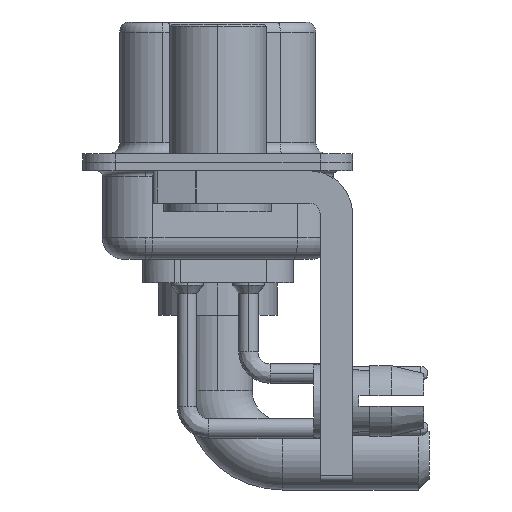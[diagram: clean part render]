
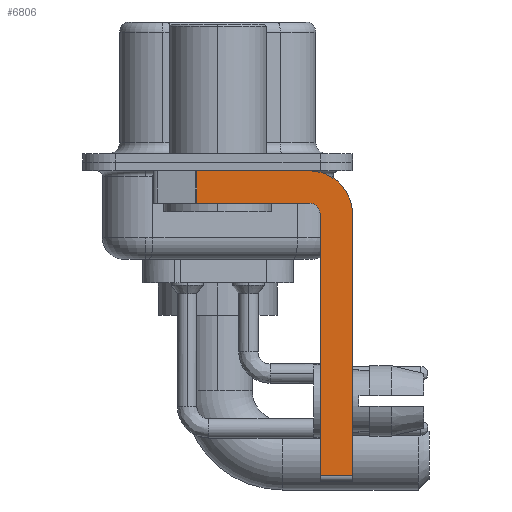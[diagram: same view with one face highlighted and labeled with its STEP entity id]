
A CAD part, left-side view. The second image highlights one B-rep face of the part: STEP entity #6806.
In plain terms, the highlighted planar face has unit normal (-1, 0, 0).
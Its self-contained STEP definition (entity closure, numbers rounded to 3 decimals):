
#232 = VERTEX_POINT ( 'NONE', #6532 ) ;
#1217 = CARTESIAN_POINT ( 'NONE',  ( -2.9, -4.75, -14.55 ) ) ;
#1303 = ORIENTED_EDGE ( 'NONE', *, *, #18957, .F. ) ;
#2598 = VERTEX_POINT ( 'NONE', #21329 ) ;
#3420 = LINE ( 'NONE', #29053, #27562 ) ;
#3523 = VECTOR ( 'NONE', #29938, 1000. ) ;
#3868 = DIRECTION ( 'NONE',  ( 0., 0., -1. ) ) ;
#3941 = DIRECTION ( 'NONE',  ( 0., 0., -1. ) ) ;
#4054 = DIRECTION ( 'NONE',  ( 1., 0., 0. ) ) ;
#4432 = LINE ( 'NONE', #11294, #3523 ) ;
#4617 = VECTOR ( 'NONE', #25354, 1000. ) ;
#4645 = CARTESIAN_POINT ( 'NONE',  ( -2.9, -4.25, -2.4 ) ) ;
#5770 = CARTESIAN_POINT ( 'NONE',  ( -2.9, -4.25, -2.4 ) ) ;
#5976 = AXIS2_PLACEMENT_3D ( 'NONE', #7387, #16223, #16380 ) ;
#6434 = EDGE_CURVE ( 'NONE', #29442, #24426, #17389, .T. ) ;
#6532 = CARTESIAN_POINT ( 'NONE',  ( -2.9, -4.25, -1.9 ) ) ;
#6806 = ADVANCED_FACE ( 'NONE', ( #10334 ), #15063, .F. ) ;
#6948 = VECTOR ( 'NONE', #23942, 1000. ) ;
#7024 = EDGE_CURVE ( 'NONE', #28893, #24217, #20632, .T. ) ;
#7387 = CARTESIAN_POINT ( 'NONE',  ( -2.9, -4.25, -2.4 ) ) ;
#8292 = ORIENTED_EDGE ( 'NONE', *, *, #28076, .F. ) ;
#9738 = ORIENTED_EDGE ( 'NONE', *, *, #29828, .T. ) ;
#9812 = ORIENTED_EDGE ( 'NONE', *, *, #18175, .F. ) ;
#10198 = EDGE_CURVE ( 'NONE', #14357, #15229, #3420, .T. ) ;
#10319 = ORIENTED_EDGE ( 'NONE', *, *, #6434, .F. ) ;
#10334 = FACE_OUTER_BOUND ( 'NONE', #21646, .T. ) ;
#10677 = CARTESIAN_POINT ( 'NONE',  ( -2.9, -4.75, -14.8 ) ) ;
#11294 = CARTESIAN_POINT ( 'NONE',  ( -2.9, -4.25, -1.9 ) ) ;
#12267 = CARTESIAN_POINT ( 'NONE',  ( -2.9, 3., -0.4 ) ) ;
#12476 = DIRECTION ( 'NONE',  ( 1., 0., 0. ) ) ;
#12500 = ORIENTED_EDGE ( 'NONE', *, *, #10198, .T. ) ;
#12681 = CARTESIAN_POINT ( 'NONE',  ( -2.9, 0.978, -0.4 ) ) ;
#14004 = CARTESIAN_POINT ( 'NONE',  ( -2.9, -4.75, -2.4 ) ) ;
#14151 = CARTESIAN_POINT ( 'NONE',  ( -2.9, 0.978, -1.9 ) ) ;
#14357 = VERTEX_POINT ( 'NONE', #12681 ) ;
#15063 = PLANE ( 'NONE',  #19733 ) ;
#15229 = VERTEX_POINT ( 'NONE', #14151 ) ;
#16108 = CARTESIAN_POINT ( 'NONE',  ( -2.9, -4.25, -14.55 ) ) ;
#16223 = DIRECTION ( 'NONE',  ( -1., 0., 0. ) ) ;
#16370 = ORIENTED_EDGE ( 'NONE', *, *, #7024, .F. ) ;
#16380 = DIRECTION ( 'NONE',  ( 0., 0., 1. ) ) ;
#17389 = LINE ( 'NONE', #10677, #26960 ) ;
#17644 = CIRCLE ( 'NONE', #5976, 0.5 ) ;
#17676 = DIRECTION ( 'NONE',  ( 0., 0., 1. ) ) ;
#17937 = CARTESIAN_POINT ( 'NONE',  ( -2.9, -6.25, -2.4 ) ) ;
#18000 = EDGE_CURVE ( 'NONE', #24426, #232, #17644, .T. ) ;
#18175 = EDGE_CURVE ( 'NONE', #14357, #2598, #19084, .T. ) ;
#18447 = CIRCLE ( 'NONE', #26194, 2. ) ;
#18957 = EDGE_CURVE ( 'NONE', #232, #15229, #4432, .T. ) ;
#19084 = LINE ( 'NONE', #12267, #6948 ) ;
#19733 = AXIS2_PLACEMENT_3D ( 'NONE', #5770, #12476, #22015 ) ;
#20046 = ORIENTED_EDGE ( 'NONE', *, *, #18000, .F. ) ;
#20632 = LINE ( 'NONE', #17937, #29896 ) ;
#20640 = CARTESIAN_POINT ( 'NONE',  ( -2.9, -6.25, -2.4 ) ) ;
#21329 = CARTESIAN_POINT ( 'NONE',  ( -2.9, -4.25, -0.4 ) ) ;
#21646 = EDGE_LOOP ( 'NONE', ( #9812, #12500, #1303, #20046, #10319, #9738, #16370, #8292 ) ) ;
#22015 = DIRECTION ( 'NONE',  ( 0., 0., -1. ) ) ;
#23070 = LINE ( 'NONE', #16108, #4617 ) ;
#23942 = DIRECTION ( 'NONE',  ( 0., -1., 0. ) ) ;
#24217 = VERTEX_POINT ( 'NONE', #27176 ) ;
#24426 = VERTEX_POINT ( 'NONE', #14004 ) ;
#25354 = DIRECTION ( 'NONE',  ( 0., -1., 0. ) ) ;
#26194 = AXIS2_PLACEMENT_3D ( 'NONE', #4645, #4054, #29847 ) ;
#26960 = VECTOR ( 'NONE', #17676, 1000. ) ;
#27176 = CARTESIAN_POINT ( 'NONE',  ( -2.9, -6.25, -14.55 ) ) ;
#27562 = VECTOR ( 'NONE', #3868, 1000. ) ;
#28076 = EDGE_CURVE ( 'NONE', #2598, #28893, #18447, .T. ) ;
#28893 = VERTEX_POINT ( 'NONE', #20640 ) ;
#29053 = CARTESIAN_POINT ( 'NONE',  ( -2.9, 0.978, -1.9 ) ) ;
#29442 = VERTEX_POINT ( 'NONE', #1217 ) ;
#29828 = EDGE_CURVE ( 'NONE', #29442, #24217, #23070, .T. ) ;
#29847 = DIRECTION ( 'NONE',  ( 0., 0., -1. ) ) ;
#29896 = VECTOR ( 'NONE', #3941, 1000. ) ;
#29938 = DIRECTION ( 'NONE',  ( 0., 1., 0. ) ) ;
